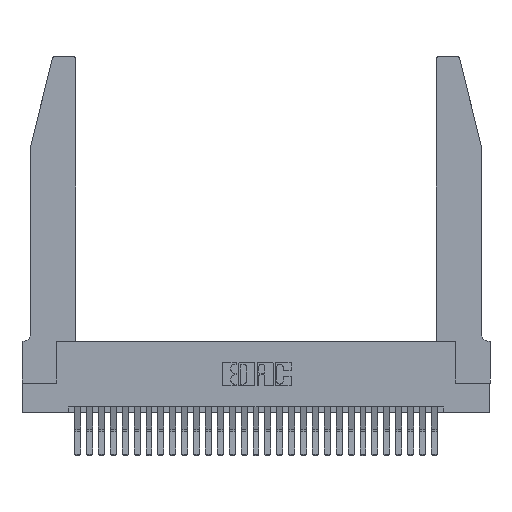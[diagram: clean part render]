
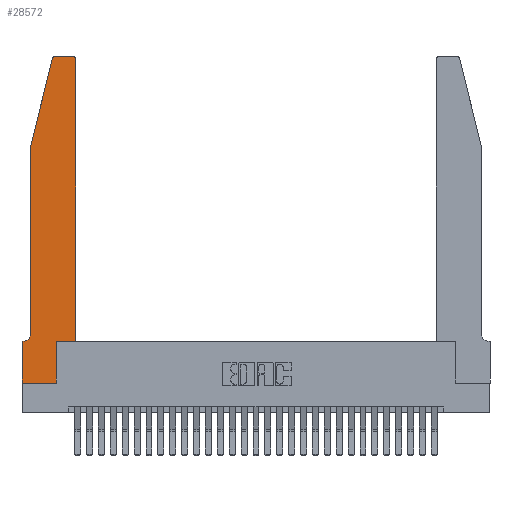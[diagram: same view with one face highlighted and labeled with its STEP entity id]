
A CAD part, top view. The second image highlights one B-rep face of the part: STEP entity #28572.
In plain terms, the highlighted planar face has unit normal (0, 0, 1).
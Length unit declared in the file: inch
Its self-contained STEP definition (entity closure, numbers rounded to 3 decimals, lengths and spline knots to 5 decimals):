
#72 = CIRCLE ( 'NONE', #2273, 0.03 ) ;
#151 = VERTEX_POINT ( 'NONE', #16935 ) ;
#276 = EDGE_CURVE ( 'NONE', #15556, #6445, #25644, .T. ) ;
#863 = VERTEX_POINT ( 'NONE', #6083 ) ;
#1348 = ORIENTED_EDGE ( 'NONE', *, *, #19645, .T. ) ;
#1724 = DIRECTION ( 'NONE',  ( -0.239, -0.971, 0. ) ) ;
#1959 = ORIENTED_EDGE ( 'NONE', *, *, #4514, .T. ) ;
#2012 = EDGE_CURVE ( 'NONE', #863, #9895, #22236, .T. ) ;
#2133 = AXIS2_PLACEMENT_3D ( 'NONE', #4478, #21164, #6884 ) ;
#2169 = AXIS2_PLACEMENT_3D ( 'NONE', #3995, #20695, #6405 ) ;
#2190 = CARTESIAN_POINT ( 'NONE',  ( 0., 0.35, 0.37 ) ) ;
#2209 = AXIS2_PLACEMENT_3D ( 'NONE', #20578, #6280, #22908 ) ;
#2273 = AXIS2_PLACEMENT_3D ( 'NONE', #23119, #8895, #25484 ) ;
#2465 = VERTEX_POINT ( 'NONE', #5984 ) ;
#2882 = CARTESIAN_POINT ( 'NONE',  ( 0., 0., 0.37 ) ) ;
#3089 = EDGE_CURVE ( 'NONE', #4930, #863, #18309, .T. ) ;
#3995 = CARTESIAN_POINT ( 'NONE',  ( 0.4205, 2.72, 0.37 ) ) ;
#4461 = EDGE_LOOP ( 'NONE', ( #6178, #7039, #18535, #30381, #1959, #28578, #1348, #18939, #18571, #11434, #14611, #17408 ) ) ;
#4478 = CARTESIAN_POINT ( 'NONE',  ( 0., 0.35, 0.37 ) ) ;
#4514 = EDGE_CURVE ( 'NONE', #2465, #15556, #18223, .T. ) ;
#4652 = VECTOR ( 'NONE', #22543, 39.37008 ) ;
#4930 = VERTEX_POINT ( 'NONE', #7613 ) ;
#5421 = LINE ( 'NONE', #11697, #23638 ) ;
#5984 = CARTESIAN_POINT ( 'NONE',  ( 0.0755, 0.42, 0.37 ) ) ;
#6083 = CARTESIAN_POINT ( 'NONE',  ( 0.4505, 0.35, 0.37 ) ) ;
#6178 = ORIENTED_EDGE ( 'NONE', *, *, #18830, .T. ) ;
#6280 = DIRECTION ( 'NONE',  ( 0., 0., -1. ) ) ;
#6326 = CARTESIAN_POINT ( 'NONE',  ( 0.2865, 0., 0.37 ) ) ;
#6405 = DIRECTION ( 'NONE',  ( 1., 0., 0. ) ) ;
#6445 = VERTEX_POINT ( 'NONE', #2190 ) ;
#6465 = CARTESIAN_POINT ( 'NONE',  ( 0.0755, 2., 0.37 ) ) ;
#6884 = DIRECTION ( 'NONE',  ( 1., 0., 0. ) ) ;
#7039 = ORIENTED_EDGE ( 'NONE', *, *, #13505, .T. ) ;
#7604 = VECTOR ( 'NONE', #21945, 39.37008 ) ;
#7613 = CARTESIAN_POINT ( 'NONE',  ( 0.2865, 0.35, 0.37 ) ) ;
#8895 = DIRECTION ( 'NONE',  ( 0., 0., 1. ) ) ;
#9604 = VERTEX_POINT ( 'NONE', #11023 ) ;
#9814 = CARTESIAN_POINT ( 'NONE',  ( 0.0755, 0.35, 0.37 ) ) ;
#9895 = VERTEX_POINT ( 'NONE', #16664 ) ;
#10547 = DIRECTION ( 'NONE',  ( 1., 0., 0. ) ) ;
#10686 = VECTOR ( 'NONE', #1724, 39.37008 ) ;
#11023 = CARTESIAN_POINT ( 'NONE',  ( 0.25487, 2.72718, 0.37 ) ) ;
#11204 = CARTESIAN_POINT ( 'NONE',  ( 0.0055, 0.35, 0.37 ) ) ;
#11227 = EDGE_CURVE ( 'NONE', #14410, #2465, #28072, .T. ) ;
#11424 = LINE ( 'NONE', #6465, #10686 ) ;
#11434 = ORIENTED_EDGE ( 'NONE', *, *, #3089, .T. ) ;
#11697 = CARTESIAN_POINT ( 'NONE',  ( 0.2605, 2.75, 0.37 ) ) ;
#12101 = EDGE_CURVE ( 'NONE', #9604, #14410, #11424, .T. ) ;
#12313 = VECTOR ( 'NONE', #12315, 39.37008 ) ;
#12315 = DIRECTION ( 'NONE',  ( -1., 0., 0. ) ) ;
#12936 = CARTESIAN_POINT ( 'NONE',  ( 0.4505, 0.35, 0.37 ) ) ;
#13505 = EDGE_CURVE ( 'NONE', #26273, #9604, #72, .T. ) ;
#13963 = CIRCLE ( 'NONE', #2169, 0.03 ) ;
#14142 = DIRECTION ( 'NONE',  ( -1., 0., 0. ) ) ;
#14205 = DIRECTION ( 'NONE',  ( 0., 1., 0. ) ) ;
#14410 = VERTEX_POINT ( 'NONE', #19307 ) ;
#14611 = ORIENTED_EDGE ( 'NONE', *, *, #2012, .T. ) ;
#15500 = LINE ( 'NONE', #2882, #7604 ) ;
#15556 = VERTEX_POINT ( 'NONE', #11204 ) ;
#15970 = VECTOR ( 'NONE', #14205, 39.37008 ) ;
#15996 = VECTOR ( 'NONE', #27070, 39.37008 ) ;
#16664 = CARTESIAN_POINT ( 'NONE',  ( 0.4505, 2.72, 0.37 ) ) ;
#16935 = CARTESIAN_POINT ( 'NONE',  ( 0.4205, 2.75, 0.37 ) ) ;
#17357 = LINE ( 'NONE', #20219, #4652 ) ;
#17408 = ORIENTED_EDGE ( 'NONE', *, *, #20160, .T. ) ;
#17561 = CARTESIAN_POINT ( 'NONE',  ( 0.2865, 0.35, 0.37 ) ) ;
#17570 = FACE_OUTER_BOUND ( 'NONE', #4461, .T. ) ;
#18223 = CIRCLE ( 'NONE', #2209, 0.07 ) ;
#18309 = LINE ( 'NONE', #29251, #23820 ) ;
#18535 = ORIENTED_EDGE ( 'NONE', *, *, #12101, .T. ) ;
#18571 = ORIENTED_EDGE ( 'NONE', *, *, #24989, .T. ) ;
#18830 = EDGE_CURVE ( 'NONE', #151, #26273, #5421, .T. ) ;
#18901 = VERTEX_POINT ( 'NONE', #19107 ) ;
#18939 = ORIENTED_EDGE ( 'NONE', *, *, #26748, .T. ) ;
#19107 = CARTESIAN_POINT ( 'NONE',  ( 0., 0., 0.37 ) ) ;
#19307 = CARTESIAN_POINT ( 'NONE',  ( 0.0755, 2., 0.37 ) ) ;
#19645 = EDGE_CURVE ( 'NONE', #6445, #18901, #15500, .T. ) ;
#20092 = DIRECTION ( 'NONE',  ( 0., -1., 0. ) ) ;
#20160 = EDGE_CURVE ( 'NONE', #9895, #151, #13963, .T. ) ;
#20219 = CARTESIAN_POINT ( 'NONE',  ( 0., 0., 0.37 ) ) ;
#20578 = CARTESIAN_POINT ( 'NONE',  ( 0.0055, 0.42, 0.37 ) ) ;
#20695 = DIRECTION ( 'NONE',  ( 0., 0., 1. ) ) ;
#21164 = DIRECTION ( 'NONE',  ( 0., 0., 1. ) ) ;
#21945 = DIRECTION ( 'NONE',  ( 0., -1., 0. ) ) ;
#22236 = LINE ( 'NONE', #12936, #15970 ) ;
#22416 = CARTESIAN_POINT ( 'NONE',  ( 0.0755, 2., 0.37 ) ) ;
#22543 = DIRECTION ( 'NONE',  ( 1., 0., 0. ) ) ;
#22575 = LINE ( 'NONE', #17561, #15996 ) ;
#22908 = DIRECTION ( 'NONE',  ( -1., 0., 0. ) ) ;
#23119 = CARTESIAN_POINT ( 'NONE',  ( 0.284, 2.72, 0.37 ) ) ;
#23638 = VECTOR ( 'NONE', #14142, 39.37008 ) ;
#23820 = VECTOR ( 'NONE', #10547, 39.37008 ) ;
#24989 = EDGE_CURVE ( 'NONE', #26874, #4930, #22575, .T. ) ;
#25484 = DIRECTION ( 'NONE',  ( 1., 0., 0. ) ) ;
#25644 = LINE ( 'NONE', #9814, #12313 ) ;
#26273 = VERTEX_POINT ( 'NONE', #29451 ) ;
#26748 = EDGE_CURVE ( 'NONE', #18901, #26874, #17357, .T. ) ;
#26874 = VERTEX_POINT ( 'NONE', #6326 ) ;
#27070 = DIRECTION ( 'NONE',  ( 0., 1., 0. ) ) ;
#27342 = VECTOR ( 'NONE', #20092, 39.37008 ) ;
#28072 = LINE ( 'NONE', #22416, #27342 ) ;
#28572 = ADVANCED_FACE ( 'NONE', ( #17570 ), #30358, .T. ) ;
#28578 = ORIENTED_EDGE ( 'NONE', *, *, #276, .T. ) ;
#29251 = CARTESIAN_POINT ( 'NONE',  ( 0.4505, 0.35, 0.37 ) ) ;
#29451 = CARTESIAN_POINT ( 'NONE',  ( 0.284, 2.75, 0.37 ) ) ;
#30358 = PLANE ( 'NONE',  #2133 ) ;
#30381 = ORIENTED_EDGE ( 'NONE', *, *, #11227, .T. ) ;
